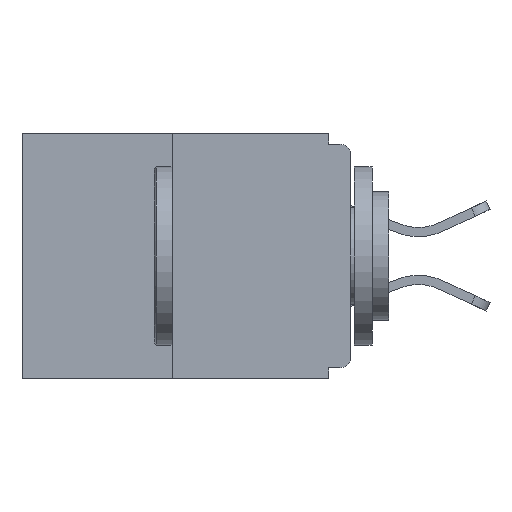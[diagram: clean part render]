
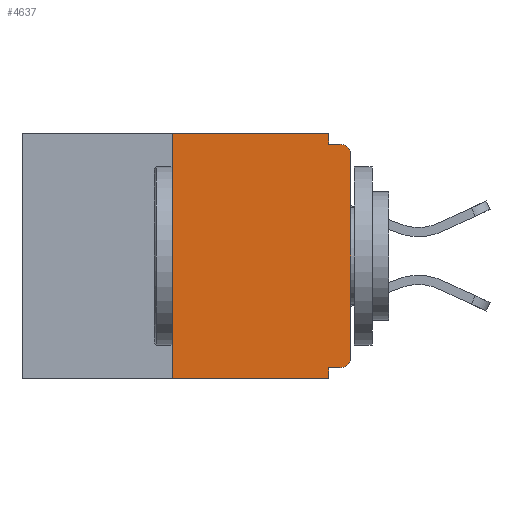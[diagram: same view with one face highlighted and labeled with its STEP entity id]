
A CAD part, left-side view. The second image highlights one B-rep face of the part: STEP entity #4637.
In plain terms, the highlighted planar face has unit normal (-1, 0, 0).
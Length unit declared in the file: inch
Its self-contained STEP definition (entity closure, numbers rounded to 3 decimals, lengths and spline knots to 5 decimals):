
#136 = EDGE_CURVE ( 'NONE', #5781, #4517, #4705, .T. ) ;
#362 = VECTOR ( 'NONE', #8929, 39.37008 ) ;
#470 = CARTESIAN_POINT ( 'NONE',  ( 0., 0., -0.015 ) ) ;
#533 = EDGE_LOOP ( 'NONE', ( #11915, #12445, #8153, #795, #12844, #8625, #10449, #6963, #3075, #11579 ) ) ;
#600 = VECTOR ( 'NONE', #3890, 39.37008 ) ;
#795 = ORIENTED_EDGE ( 'NONE', *, *, #136, .F. ) ;
#932 = VERTEX_POINT ( 'NONE', #3916 ) ;
#1061 = EDGE_CURVE ( 'NONE', #932, #7758, #5119, .T. ) ;
#1399 = EDGE_CURVE ( 'NONE', #11991, #7758, #12569, .T. ) ;
#1413 = LINE ( 'NONE', #12413, #10600 ) ;
#1471 = VECTOR ( 'NONE', #10098, 39.37008 ) ;
#1774 = VECTOR ( 'NONE', #12536, 39.37008 ) ;
#1788 = CARTESIAN_POINT ( 'NONE',  ( 0., 0., -0.03 ) ) ;
#1939 = CARTESIAN_POINT ( 'NONE',  ( 0., 0.015, -0.313 ) ) ;
#2044 = CARTESIAN_POINT ( 'NONE',  ( 0., 0.015, -0.328 ) ) ;
#2275 = CARTESIAN_POINT ( 'NONE',  ( 0., 0.25, 0. ) ) ;
#2435 = CARTESIAN_POINT ( 'NONE',  ( 0., 0.015, -0.03 ) ) ;
#2505 = LINE ( 'NONE', #9410, #7257 ) ;
#2665 = FACE_OUTER_BOUND ( 'NONE', #533, .T. ) ;
#2896 = AXIS2_PLACEMENT_3D ( 'NONE', #1939, #4029, #9059 ) ;
#3075 = ORIENTED_EDGE ( 'NONE', *, *, #1061, .F. ) ;
#3890 = DIRECTION ( 'NONE',  ( 0., 0., 1. ) ) ;
#3916 = CARTESIAN_POINT ( 'NONE',  ( 0., 0.031, -0.015 ) ) ;
#3973 = CARTESIAN_POINT ( 'NONE',  ( 0., 0.25, 0. ) ) ;
#3991 = EDGE_CURVE ( 'NONE', #7772, #7420, #7099, .T. ) ;
#4029 = DIRECTION ( 'NONE',  ( -1., 0., 0. ) ) ;
#4156 = CARTESIAN_POINT ( 'NONE',  ( 0., 0., -0.313 ) ) ;
#4243 = EDGE_CURVE ( 'NONE', #5448, #4517, #1413, .T. ) ;
#4399 = CARTESIAN_POINT ( 'NONE',  ( 0., 0.46, 0. ) ) ;
#4502 = VECTOR ( 'NONE', #12523, 39.37008 ) ;
#4517 = VERTEX_POINT ( 'NONE', #5521 ) ;
#4637 = ADVANCED_FACE ( 'NONE', ( #2665 ), #7251, .F. ) ;
#4677 = LINE ( 'NONE', #10528, #4502 ) ;
#4705 = LINE ( 'NONE', #6178, #11324 ) ;
#4738 = LINE ( 'NONE', #3973, #600 ) ;
#5082 = CARTESIAN_POINT ( 'NONE',  ( 0., 0.031, 0. ) ) ;
#5119 = LINE ( 'NONE', #470, #362 ) ;
#5135 = CARTESIAN_POINT ( 'NONE',  ( 0., 0.015, -0.015 ) ) ;
#5171 = AXIS2_PLACEMENT_3D ( 'NONE', #2435, #10677, #7565 ) ;
#5448 = VERTEX_POINT ( 'NONE', #6362 ) ;
#5477 = DIRECTION ( 'NONE',  ( 0., 0., -1. ) ) ;
#5491 = CARTESIAN_POINT ( 'NONE',  ( 0., 0.031, -0.328 ) ) ;
#5521 = CARTESIAN_POINT ( 'NONE',  ( 0., 0.031, -0.343 ) ) ;
#5660 = EDGE_CURVE ( 'NONE', #7772, #5781, #4677, .T. ) ;
#5781 = VERTEX_POINT ( 'NONE', #5491 ) ;
#5936 = VERTEX_POINT ( 'NONE', #2275 ) ;
#6178 = CARTESIAN_POINT ( 'NONE',  ( 0., 0.031, -0.343 ) ) ;
#6362 = CARTESIAN_POINT ( 'NONE',  ( 0., 0.25, -0.343 ) ) ;
#6407 = CARTESIAN_POINT ( 'NONE',  ( 0., 0.031, 0. ) ) ;
#6963 = ORIENTED_EDGE ( 'NONE', *, *, #1399, .T. ) ;
#7099 = CIRCLE ( 'NONE', #2896, 0.015 ) ;
#7251 = PLANE ( 'NONE',  #9820 ) ;
#7257 = VECTOR ( 'NONE', #7345, 39.37008 ) ;
#7261 = EDGE_CURVE ( 'NONE', #7420, #11991, #8891, .T. ) ;
#7343 = DIRECTION ( 'NONE',  ( 1., 0., 0. ) ) ;
#7345 = DIRECTION ( 'NONE',  ( 0., -1., 0. ) ) ;
#7420 = VERTEX_POINT ( 'NONE', #4156 ) ;
#7562 = CARTESIAN_POINT ( 'NONE',  ( 0., 0., 0. ) ) ;
#7565 = DIRECTION ( 'NONE',  ( 0., 0., -1. ) ) ;
#7758 = VERTEX_POINT ( 'NONE', #5135 ) ;
#7772 = VERTEX_POINT ( 'NONE', #2044 ) ;
#8153 = ORIENTED_EDGE ( 'NONE', *, *, #4243, .T. ) ;
#8264 = DIRECTION ( 'NONE',  ( 0., 0., -1. ) ) ;
#8422 = DIRECTION ( 'NONE',  ( 0., -1., 0. ) ) ;
#8595 = LINE ( 'NONE', #5082, #1471 ) ;
#8625 = ORIENTED_EDGE ( 'NONE', *, *, #3991, .T. ) ;
#8737 = EDGE_CURVE ( 'NONE', #5936, #11874, #2505, .T. ) ;
#8891 = LINE ( 'NONE', #7562, #1774 ) ;
#8929 = DIRECTION ( 'NONE',  ( 0., -1., 0. ) ) ;
#9059 = DIRECTION ( 'NONE',  ( 0., 0., -1. ) ) ;
#9410 = CARTESIAN_POINT ( 'NONE',  ( 0., 0.46, 0. ) ) ;
#9414 = EDGE_CURVE ( 'NONE', #5448, #5936, #4738, .T. ) ;
#9820 = AXIS2_PLACEMENT_3D ( 'NONE', #4399, #7343, #8264 ) ;
#10098 = DIRECTION ( 'NONE',  ( 0., 0., -1. ) ) ;
#10449 = ORIENTED_EDGE ( 'NONE', *, *, #7261, .T. ) ;
#10528 = CARTESIAN_POINT ( 'NONE',  ( 0., 0., -0.328 ) ) ;
#10600 = VECTOR ( 'NONE', #8422, 39.37008 ) ;
#10677 = DIRECTION ( 'NONE',  ( -1., 0., 0. ) ) ;
#11324 = VECTOR ( 'NONE', #5477, 39.37008 ) ;
#11579 = ORIENTED_EDGE ( 'NONE', *, *, #12044, .F. ) ;
#11874 = VERTEX_POINT ( 'NONE', #6407 ) ;
#11915 = ORIENTED_EDGE ( 'NONE', *, *, #8737, .F. ) ;
#11991 = VERTEX_POINT ( 'NONE', #1788 ) ;
#12044 = EDGE_CURVE ( 'NONE', #11874, #932, #8595, .T. ) ;
#12413 = CARTESIAN_POINT ( 'NONE',  ( 0., 0.46, -0.343 ) ) ;
#12445 = ORIENTED_EDGE ( 'NONE', *, *, #9414, .F. ) ;
#12523 = DIRECTION ( 'NONE',  ( 0., 1., 0. ) ) ;
#12536 = DIRECTION ( 'NONE',  ( 0., 0., 1. ) ) ;
#12569 = CIRCLE ( 'NONE', #5171, 0.015 ) ;
#12844 = ORIENTED_EDGE ( 'NONE', *, *, #5660, .F. ) ;
